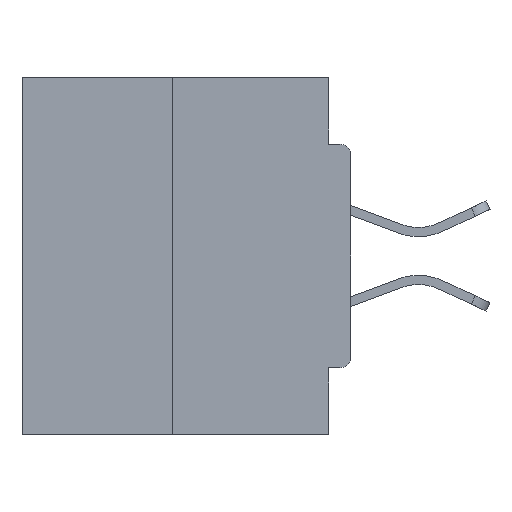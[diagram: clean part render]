
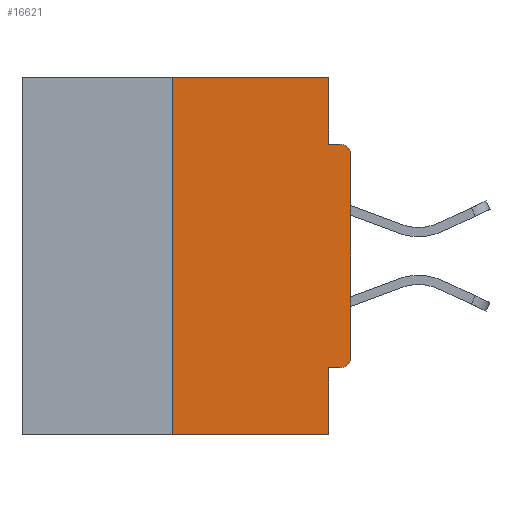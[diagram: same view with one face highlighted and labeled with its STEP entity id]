
A CAD part, left-side view. The second image highlights one B-rep face of the part: STEP entity #16621.
In plain terms, the highlighted planar face has unit normal (-1, 0, 0).
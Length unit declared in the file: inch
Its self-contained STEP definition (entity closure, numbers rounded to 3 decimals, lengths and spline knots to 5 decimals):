
#635 = LINE ( 'NONE', #34004, #11957 ) ;
#1433 = EDGE_CURVE ( 'NONE', #4400, #21222, #24124, .T. ) ;
#1550 = LINE ( 'NONE', #5996, #14968 ) ;
#1624 = DIRECTION ( 'NONE',  ( 0., -1., 0. ) ) ;
#2141 = CIRCLE ( 'NONE', #13052, 0.015 ) ;
#2605 = DIRECTION ( 'NONE',  ( 0., -1., 0. ) ) ;
#2757 = LINE ( 'NONE', #15840, #16566 ) ;
#2994 = ORIENTED_EDGE ( 'NONE', *, *, #20305, .F. ) ;
#3235 = ORIENTED_EDGE ( 'NONE', *, *, #12922, .F. ) ;
#4400 = VERTEX_POINT ( 'NONE', #25114 ) ;
#4746 = ORIENTED_EDGE ( 'NONE', *, *, #20858, .T. ) ;
#5579 = ORIENTED_EDGE ( 'NONE', *, *, #11855, .F. ) ;
#5657 = EDGE_CURVE ( 'NONE', #17775, #4400, #7961, .T. ) ;
#5721 = ORIENTED_EDGE ( 'NONE', *, *, #11335, .F. ) ;
#5996 = CARTESIAN_POINT ( 'NONE',  ( 0., 0.031, -0.5 ) ) ;
#6739 = ORIENTED_EDGE ( 'NONE', *, *, #24088, .T. ) ;
#7343 = CARTESIAN_POINT ( 'NONE',  ( 0., 0., 0. ) ) ;
#7961 = LINE ( 'NONE', #7343, #16705 ) ;
#8151 = CARTESIAN_POINT ( 'NONE',  ( 0., 0.031, 0. ) ) ;
#8689 = CARTESIAN_POINT ( 'NONE',  ( 0., 0.031, -0.0935 ) ) ;
#8776 = DIRECTION ( 'NONE',  ( 0., 0., -1. ) ) ;
#9244 = FACE_OUTER_BOUND ( 'NONE', #13978, .T. ) ;
#9345 = CARTESIAN_POINT ( 'NONE',  ( 0., 0.25, 0. ) ) ;
#9398 = LINE ( 'NONE', #9345, #32369 ) ;
#9487 = VERTEX_POINT ( 'NONE', #8689 ) ;
#10345 = ORIENTED_EDGE ( 'NONE', *, *, #1433, .T. ) ;
#10421 = CARTESIAN_POINT ( 'NONE',  ( 0., 0.015, -0.0935 ) ) ;
#10847 = CARTESIAN_POINT ( 'NONE',  ( 0., 0., -0.3915 ) ) ;
#11335 = EDGE_CURVE ( 'NONE', #9487, #21222, #635, .T. ) ;
#11769 = VERTEX_POINT ( 'NONE', #23806 ) ;
#11855 = EDGE_CURVE ( 'NONE', #20945, #9487, #20738, .T. ) ;
#11957 = VECTOR ( 'NONE', #18949, 39.37008 ) ;
#12314 = CARTESIAN_POINT ( 'NONE',  ( 0., 0.25, 0. ) ) ;
#12742 = CARTESIAN_POINT ( 'NONE',  ( 0., 0.46, 0. ) ) ;
#12791 = AXIS2_PLACEMENT_3D ( 'NONE', #12742, #15458, #8776 ) ;
#12922 = EDGE_CURVE ( 'NONE', #11769, #14150, #31925, .T. ) ;
#13052 = AXIS2_PLACEMENT_3D ( 'NONE', #18473, #13435, #31871 ) ;
#13158 = DIRECTION ( 'NONE',  ( 0., 0., -1. ) ) ;
#13435 = DIRECTION ( 'NONE',  ( -1., 0., 0. ) ) ;
#13905 = EDGE_CURVE ( 'NONE', #23984, #14572, #9398, .T. ) ;
#13978 = EDGE_LOOP ( 'NONE', ( #26581, #24302, #4746, #2994, #3235, #6739, #33159, #10345, #5721, #5579 ) ) ;
#14150 = VERTEX_POINT ( 'NONE', #31267 ) ;
#14183 = DIRECTION ( 'NONE',  ( 0., 0., -1. ) ) ;
#14572 = VERTEX_POINT ( 'NONE', #12314 ) ;
#14642 = CARTESIAN_POINT ( 'NONE',  ( 0., 0.031, 0. ) ) ;
#14968 = VECTOR ( 'NONE', #14183, 39.37008 ) ;
#15458 = DIRECTION ( 'NONE',  ( 1., 0., 0. ) ) ;
#15840 = CARTESIAN_POINT ( 'NONE',  ( 0., 0.46, -0.5 ) ) ;
#16059 = VECTOR ( 'NONE', #21286, 39.37008 ) ;
#16566 = VECTOR ( 'NONE', #2605, 39.37008 ) ;
#16621 = ADVANCED_FACE ( 'NONE', ( #9244 ), #25821, .F. ) ;
#16705 = VECTOR ( 'NONE', #29035, 39.37008 ) ;
#17000 = VECTOR ( 'NONE', #13158, 39.37008 ) ;
#17314 = CARTESIAN_POINT ( 'NONE',  ( 0., 0.015, -0.1085 ) ) ;
#17430 = AXIS2_PLACEMENT_3D ( 'NONE', #17314, #25793, #17556 ) ;
#17556 = DIRECTION ( 'NONE',  ( 0., 0., -1. ) ) ;
#17775 = VERTEX_POINT ( 'NONE', #10847 ) ;
#18473 = CARTESIAN_POINT ( 'NONE',  ( 0., 0.015, -0.3915 ) ) ;
#18949 = DIRECTION ( 'NONE',  ( 0., -1., 0. ) ) ;
#20305 = EDGE_CURVE ( 'NONE', #14150, #25610, #1550, .T. ) ;
#20738 = LINE ( 'NONE', #8151, #17000 ) ;
#20858 = EDGE_CURVE ( 'NONE', #23984, #25610, #2757, .T. ) ;
#20945 = VERTEX_POINT ( 'NONE', #14642 ) ;
#21222 = VERTEX_POINT ( 'NONE', #10421 ) ;
#21286 = DIRECTION ( 'NONE',  ( 0., 1., 0. ) ) ;
#22264 = LINE ( 'NONE', #30954, #29746 ) ;
#23645 = CARTESIAN_POINT ( 'NONE',  ( 0., 0., -0.4065 ) ) ;
#23806 = CARTESIAN_POINT ( 'NONE',  ( 0., 0.015, -0.4065 ) ) ;
#23984 = VERTEX_POINT ( 'NONE', #25914 ) ;
#24088 = EDGE_CURVE ( 'NONE', #11769, #17775, #2141, .T. ) ;
#24124 = CIRCLE ( 'NONE', #17430, 0.015 ) ;
#24302 = ORIENTED_EDGE ( 'NONE', *, *, #13905, .F. ) ;
#24941 = CARTESIAN_POINT ( 'NONE',  ( 0., 0.031, -0.5 ) ) ;
#24999 = DIRECTION ( 'NONE',  ( 0., 0., 1. ) ) ;
#25114 = CARTESIAN_POINT ( 'NONE',  ( 0., 0., -0.1085 ) ) ;
#25610 = VERTEX_POINT ( 'NONE', #24941 ) ;
#25793 = DIRECTION ( 'NONE',  ( -1., 0., 0. ) ) ;
#25821 = PLANE ( 'NONE',  #12791 ) ;
#25914 = CARTESIAN_POINT ( 'NONE',  ( 0., 0.25, -0.5 ) ) ;
#26581 = ORIENTED_EDGE ( 'NONE', *, *, #26771, .F. ) ;
#26771 = EDGE_CURVE ( 'NONE', #14572, #20945, #22264, .T. ) ;
#29035 = DIRECTION ( 'NONE',  ( 0., 0., 1. ) ) ;
#29746 = VECTOR ( 'NONE', #1624, 39.37008 ) ;
#30954 = CARTESIAN_POINT ( 'NONE',  ( 0., 0.46, 0. ) ) ;
#31267 = CARTESIAN_POINT ( 'NONE',  ( 0., 0.031, -0.4065 ) ) ;
#31871 = DIRECTION ( 'NONE',  ( 0., 0., -1. ) ) ;
#31925 = LINE ( 'NONE', #23645, #16059 ) ;
#32369 = VECTOR ( 'NONE', #24999, 39.37008 ) ;
#33159 = ORIENTED_EDGE ( 'NONE', *, *, #5657, .T. ) ;
#34004 = CARTESIAN_POINT ( 'NONE',  ( 0., 0., -0.0935 ) ) ;
